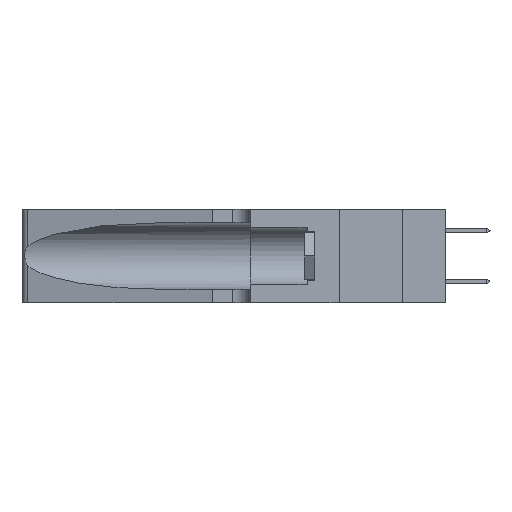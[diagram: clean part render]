
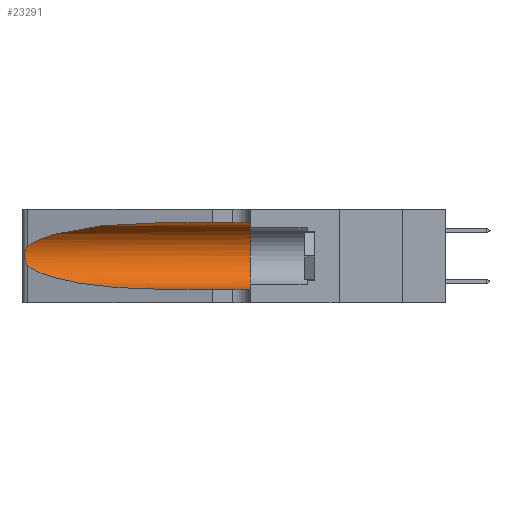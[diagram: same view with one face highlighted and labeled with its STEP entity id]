
A CAD part, left-side view. The second image highlights one B-rep face of the part: STEP entity #23291.
In plain terms, the highlighted cylindrical face has radius 3.308 mm (diameter 6.617 mm), a partial arc.
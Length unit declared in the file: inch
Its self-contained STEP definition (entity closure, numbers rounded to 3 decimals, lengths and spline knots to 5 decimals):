
#660 = DIRECTION ( 'NONE',  ( 0., -1., 0. ) ) ;
#672 =( BOUNDED_CURVE ( )  B_SPLINE_CURVE ( 3, ( #26605, #13697, #20222, #26746 ),
 .UNSPECIFIED., .F., .F. ) 
 B_SPLINE_CURVE_WITH_KNOTS ( ( 4, 4 ),
 ( 3.44316, 4.71239 ),
 .UNSPECIFIED. ) 
 CURVE ( )  GEOMETRIC_REPRESENTATION_ITEM ( )  RATIONAL_B_SPLINE_CURVE ( ( 1., 0.87, 0.87, 1. ) ) 
 REPRESENTATION_ITEM ( '' )  );
#1571 = ORIENTED_EDGE ( 'NONE', *, *, #33804, .T. ) ;
#2298 = CARTESIAN_POINT ( 'NONE',  ( 0.1305, 0.72297, 0.31525 ) ) ;
#3004 = LINE ( 'NONE', #31065, #16188 ) ;
#4164 = CARTESIAN_POINT ( 'NONE',  ( 0.26018, 1.23835, 0.19895 ) ) ;
#4553 = B_SPLINE_CURVE_WITH_KNOTS ( 'NONE', 3,
 ( #6862, #32753, #7137, #36124, #29761, #4164, #23862, #13637, #32895, #20170, #26825, #33312, #7275, #13926 ),
 .UNSPECIFIED., .F., .F.,
 ( 4, 2, 2, 2, 2, 2, 4 ),
 ( 0., 0.00027, 0.00053, 0.00107, 0.0016, 0.00187, 0.00214 ),
 .UNSPECIFIED. ) ;
#4976 = CARTESIAN_POINT ( 'NONE',  ( 0.2373, 1.15595, 0.28018 ) ) ;
#6100 = AXIS2_PLACEMENT_3D ( 'NONE', #21256, #30125, #11769 ) ;
#6605 = VERTEX_POINT ( 'NONE', #21038 ) ;
#6862 = CARTESIAN_POINT ( 'NONE',  ( 0.25487, 1.22718, 0.22369 ) ) ;
#7137 = CARTESIAN_POINT ( 'NONE',  ( 0.25639, 1.23184, 0.21858 ) ) ;
#7275 = CARTESIAN_POINT ( 'NONE',  ( 0.25555, 1.22993, 0.14849 ) ) ;
#9735 = CARTESIAN_POINT ( 'NONE',  ( 0.1305, 1.61858, 0.185 ) ) ;
#9888 = ORIENTED_EDGE ( 'NONE', *, *, #21255, .F. ) ;
#11769 = DIRECTION ( 'NONE',  ( 0., 0., 1. ) ) ;
#11782 = CARTESIAN_POINT ( 'NONE',  ( 0.25487, 1.22718, 0.22369 ) ) ;
#11791 = CARTESIAN_POINT ( 'NONE',  ( 0.25487, 1.22718, 0.22369 ) ) ;
#12123 = AXIS2_PLACEMENT_3D ( 'NONE', #9735, #38461, #16153 ) ;
#13637 = CARTESIAN_POINT ( 'NONE',  ( 0.26075, 1.23896, 0.178 ) ) ;
#13697 = CARTESIAN_POINT ( 'NONE',  ( 0.2373, 1.15595, 0.08982 ) ) ;
#13886 = VERTEX_POINT ( 'NONE', #39741 ) ;
#13893 =( BOUNDED_CURVE ( )  B_SPLINE_CURVE ( 3, ( #2298, #24949, #4976, #11782 ),
 .UNSPECIFIED., .F., .F. ) 
 B_SPLINE_CURVE_WITH_KNOTS ( ( 4, 4 ),
 ( 1.5708, 2.84003 ),
 .UNSPECIFIED. ) 
 CURVE ( )  GEOMETRIC_REPRESENTATION_ITEM ( )  RATIONAL_B_SPLINE_CURVE ( ( 1., 0.87, 0.87, 1. ) ) 
 REPRESENTATION_ITEM ( '' )  );
#13926 = CARTESIAN_POINT ( 'NONE',  ( 0.25487, 1.22718, 0.14631 ) ) ;
#14290 = EDGE_CURVE ( 'NONE', #18412, #6605, #4553, .T. ) ;
#14504 = EDGE_CURVE ( 'NONE', #24903, #13886, #20864, .T. ) ;
#14814 = ORIENTED_EDGE ( 'NONE', *, *, #40724, .F. ) ;
#16153 = DIRECTION ( 'NONE',  ( 0., 0., -1. ) ) ;
#16188 = VECTOR ( 'NONE', #17793, 39.37008 ) ;
#16807 = VECTOR ( 'NONE', #660, 39.37008 ) ;
#16976 = EDGE_CURVE ( 'NONE', #6605, #24903, #672, .T. ) ;
#17793 = DIRECTION ( 'NONE',  ( 0., -1., 0. ) ) ;
#18412 = VERTEX_POINT ( 'NONE', #11791 ) ;
#20170 = CARTESIAN_POINT ( 'NONE',  ( 0.25856, 1.23593, 0.16098 ) ) ;
#20222 = CARTESIAN_POINT ( 'NONE',  ( 0.18966, 0.96281, 0.05475 ) ) ;
#20864 = LINE ( 'NONE', #30968, #16807 ) ;
#21038 = CARTESIAN_POINT ( 'NONE',  ( 0.25487, 1.22718, 0.14631 ) ) ;
#21255 = EDGE_CURVE ( 'NONE', #41180, #13886, #35466, .T. ) ;
#21256 = CARTESIAN_POINT ( 'NONE',  ( 0.1305, 0.35, 0.185 ) ) ;
#22114 = ORIENTED_EDGE ( 'NONE', *, *, #16976, .T. ) ;
#23072 = EDGE_LOOP ( 'NONE', ( #1571, #34485, #22114, #29731, #9888, #14814 ) ) ;
#23291 = ADVANCED_FACE ( 'NONE', ( #38402 ), #25778, .F. ) ;
#23862 = CARTESIAN_POINT ( 'NONE',  ( 0.26075, 1.23896, 0.19203 ) ) ;
#24903 = VERTEX_POINT ( 'NONE', #38513 ) ;
#24949 = CARTESIAN_POINT ( 'NONE',  ( 0.18966, 0.96281, 0.31525 ) ) ;
#25778 = CYLINDRICAL_SURFACE ( 'NONE', #12123, 0.13025 ) ;
#26605 = CARTESIAN_POINT ( 'NONE',  ( 0.25487, 1.22718, 0.14631 ) ) ;
#26746 = CARTESIAN_POINT ( 'NONE',  ( 0.1305, 0.72297, 0.05475 ) ) ;
#26825 = CARTESIAN_POINT ( 'NONE',  ( 0.25789, 1.23486, 0.15765 ) ) ;
#28869 = CARTESIAN_POINT ( 'NONE',  ( 0.1305, 0.72297, 0.31525 ) ) ;
#29731 = ORIENTED_EDGE ( 'NONE', *, *, #14504, .T. ) ;
#29761 = CARTESIAN_POINT ( 'NONE',  ( 0.25854, 1.2359, 0.20912 ) ) ;
#30125 = DIRECTION ( 'NONE',  ( 0., 1., 0. ) ) ;
#30968 = CARTESIAN_POINT ( 'NONE',  ( 0.1305, 1.61858, 0.05475 ) ) ;
#31065 = CARTESIAN_POINT ( 'NONE',  ( 0.1305, 1.61858, 0.31525 ) ) ;
#32753 = CARTESIAN_POINT ( 'NONE',  ( 0.25555, 1.22994, 0.2215 ) ) ;
#32895 = CARTESIAN_POINT ( 'NONE',  ( 0.26017, 1.23833, 0.17102 ) ) ;
#33312 = CARTESIAN_POINT ( 'NONE',  ( 0.25639, 1.23186, 0.15144 ) ) ;
#33804 = EDGE_CURVE ( 'NONE', #39558, #18412, #13893, .T. ) ;
#34485 = ORIENTED_EDGE ( 'NONE', *, *, #14290, .T. ) ;
#35250 = CARTESIAN_POINT ( 'NONE',  ( 0.1305, 0.35, 0.31525 ) ) ;
#35466 = CIRCLE ( 'NONE', #6100, 0.13025 ) ;
#36124 = CARTESIAN_POINT ( 'NONE',  ( 0.25787, 1.23484, 0.2124 ) ) ;
#38402 = FACE_OUTER_BOUND ( 'NONE', #23072, .T. ) ;
#38461 = DIRECTION ( 'NONE',  ( 0., -1., 0. ) ) ;
#38513 = CARTESIAN_POINT ( 'NONE',  ( 0.1305, 0.72297, 0.05475 ) ) ;
#39558 = VERTEX_POINT ( 'NONE', #28869 ) ;
#39741 = CARTESIAN_POINT ( 'NONE',  ( 0.1305, 0.35, 0.05475 ) ) ;
#40724 = EDGE_CURVE ( 'NONE', #39558, #41180, #3004, .T. ) ;
#41180 = VERTEX_POINT ( 'NONE', #35250 ) ;
